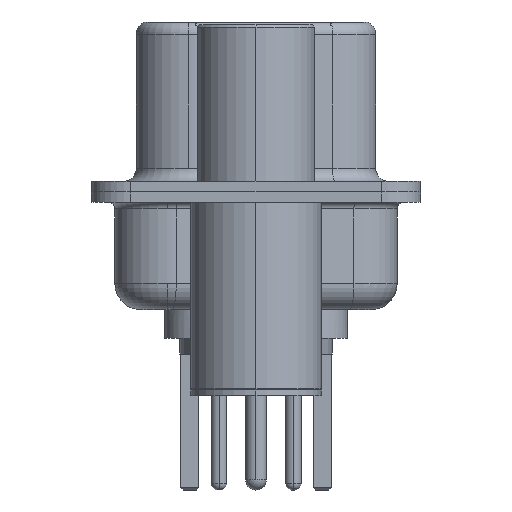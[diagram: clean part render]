
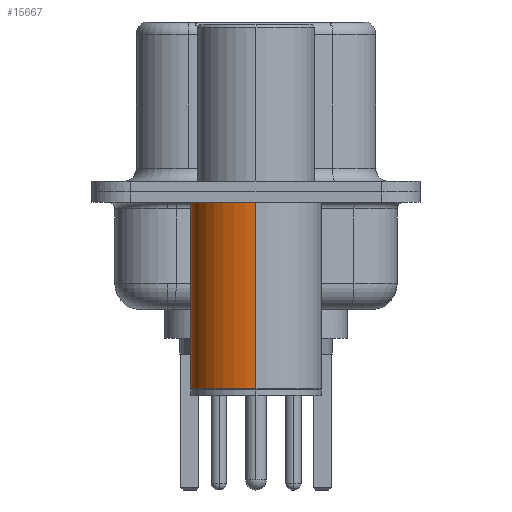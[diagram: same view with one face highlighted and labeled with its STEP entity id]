
A CAD part, left-side view. The second image highlights one B-rep face of the part: STEP entity #15667.
In plain terms, the highlighted cylindrical face has radius 2.5 mm (diameter 5 mm), a partial arc.
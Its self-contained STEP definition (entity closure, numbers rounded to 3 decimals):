
#197 = AXIS2_PLACEMENT_3D ( 'NONE', #31089, #29028, #15014 ) ;
#1793 = EDGE_LOOP ( 'NONE', ( #23822, #15017, #31839, #17403 ) ) ;
#1795 = EDGE_CURVE ( 'NONE', #27018, #28960, #17997, .T. ) ;
#2418 = CARTESIAN_POINT ( 'NONE',  ( 0., 0., 0.581 ) ) ;
#3618 = CARTESIAN_POINT ( 'NONE',  ( 2.5, 0., -7.525 ) ) ;
#4842 = LINE ( 'NONE', #23299, #10792 ) ;
#5615 = EDGE_CURVE ( 'NONE', #8991, #7440, #22840, .T. ) ;
#6801 = AXIS2_PLACEMENT_3D ( 'NONE', #2418, #7485, #22336 ) ;
#7440 = VERTEX_POINT ( 'NONE', #31056 ) ;
#7485 = DIRECTION ( 'NONE',  ( 0., 0., 1. ) ) ;
#8991 = VERTEX_POINT ( 'NONE', #14650 ) ;
#9650 = EDGE_CURVE ( 'NONE', #28960, #7440, #26062, .T. ) ;
#10792 = VECTOR ( 'NONE', #28317, 1000. ) ;
#12192 = VECTOR ( 'NONE', #19886, 1000. ) ;
#14198 = FACE_OUTER_BOUND ( 'NONE', #1793, .T. ) ;
#14650 = CARTESIAN_POINT ( 'NONE',  ( 2.5, 0., -0.4 ) ) ;
#15014 = DIRECTION ( 'NONE',  ( 1., 0., 0. ) ) ;
#15017 = ORIENTED_EDGE ( 'NONE', *, *, #9650, .T. ) ;
#15667 = ADVANCED_FACE ( 'NONE', ( #14198 ), #26542, .T. ) ;
#17032 = DIRECTION ( 'NONE',  ( 0., 0., 1. ) ) ;
#17376 = CARTESIAN_POINT ( 'NONE',  ( -2.5, 0., 0.581 ) ) ;
#17403 = ORIENTED_EDGE ( 'NONE', *, *, #30597, .F. ) ;
#17997 = CIRCLE ( 'NONE', #24017, 2.5 ) ;
#19886 = DIRECTION ( 'NONE',  ( 0., 0., 1. ) ) ;
#21163 = DIRECTION ( 'NONE',  ( 1., 0., 0. ) ) ;
#21270 = CARTESIAN_POINT ( 'NONE',  ( 0., 0., -7.525 ) ) ;
#22336 = DIRECTION ( 'NONE',  ( 1., 0., 0. ) ) ;
#22840 = CIRCLE ( 'NONE', #197, 2.5 ) ;
#23299 = CARTESIAN_POINT ( 'NONE',  ( 2.5, 0., 0.581 ) ) ;
#23822 = ORIENTED_EDGE ( 'NONE', *, *, #1795, .T. ) ;
#24017 = AXIS2_PLACEMENT_3D ( 'NONE', #21270, #17032, #21163 ) ;
#24453 = CARTESIAN_POINT ( 'NONE',  ( -2.5, 0., -7.525 ) ) ;
#26062 = LINE ( 'NONE', #17376, #12192 ) ;
#26542 = CYLINDRICAL_SURFACE ( 'NONE', #6801, 2.5 ) ;
#27018 = VERTEX_POINT ( 'NONE', #3618 ) ;
#28317 = DIRECTION ( 'NONE',  ( 0., 0., 1. ) ) ;
#28960 = VERTEX_POINT ( 'NONE', #24453 ) ;
#29028 = DIRECTION ( 'NONE',  ( 0., 0., 1. ) ) ;
#30597 = EDGE_CURVE ( 'NONE', #27018, #8991, #4842, .T. ) ;
#31056 = CARTESIAN_POINT ( 'NONE',  ( -2.5, 0., -0.4 ) ) ;
#31089 = CARTESIAN_POINT ( 'NONE',  ( 0., 0., -0.4 ) ) ;
#31839 = ORIENTED_EDGE ( 'NONE', *, *, #5615, .F. ) ;
